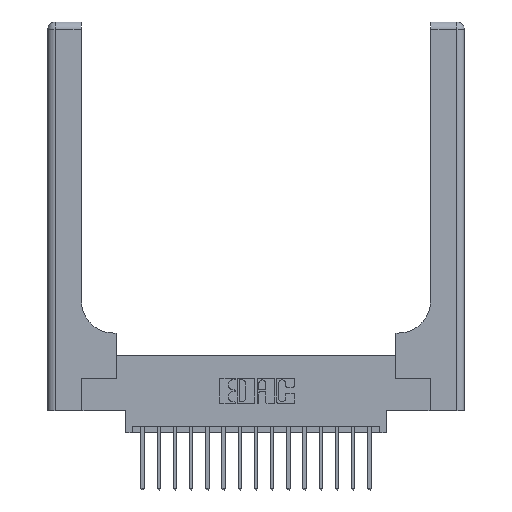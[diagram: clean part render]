
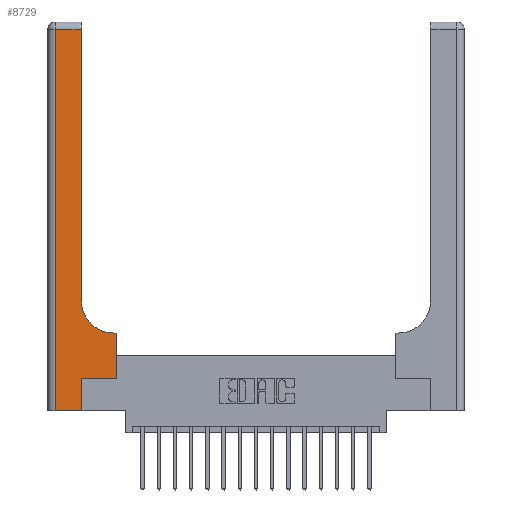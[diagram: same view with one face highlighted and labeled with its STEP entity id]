
A CAD part, top view. The second image highlights one B-rep face of the part: STEP entity #8729.
In plain terms, the highlighted planar face has unit normal (0, 0, 1).
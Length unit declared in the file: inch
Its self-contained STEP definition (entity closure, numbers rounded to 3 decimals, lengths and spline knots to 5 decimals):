
#74 = CARTESIAN_POINT ( 'NONE',  ( 0.06, 3., 0.37 ) ) ;
#119 = EDGE_CURVE ( 'NONE', #1267, #13343, #17823, .T. ) ;
#148 = DIRECTION ( 'NONE',  ( 1., 0., 0. ) ) ;
#470 = VERTEX_POINT ( 'NONE', #6315 ) ;
#1227 = VECTOR ( 'NONE', #5650, 39.37008 ) ;
#1267 = VERTEX_POINT ( 'NONE', #4174 ) ;
#1380 = ORIENTED_EDGE ( 'NONE', *, *, #119, .T. ) ;
#1852 = EDGE_CURVE ( 'NONE', #11906, #4479, #4620, .T. ) ;
#1927 = CARTESIAN_POINT ( 'NONE',  ( 0.528, 0.6, 0.37 ) ) ;
#1991 = EDGE_CURVE ( 'NONE', #9378, #11906, #12276, .T. ) ;
#2006 = CARTESIAN_POINT ( 'NONE',  ( 0.528, 0.25, 0.37 ) ) ;
#2130 = AXIS2_PLACEMENT_3D ( 'NONE', #5486, #17519, #5780 ) ;
#2336 = DIRECTION ( 'NONE',  ( -1., 0., 0. ) ) ;
#2388 = ORIENTED_EDGE ( 'NONE', *, *, #10496, .T. ) ;
#3662 = DIRECTION ( 'NONE',  ( 0., 0., -1. ) ) ;
#4174 = CARTESIAN_POINT ( 'NONE',  ( 0.06, 0., 0.37 ) ) ;
#4377 = VECTOR ( 'NONE', #17555, 39.37008 ) ;
#4388 = CARTESIAN_POINT ( 'NONE',  ( 0., 2.94, 0.37 ) ) ;
#4479 = VERTEX_POINT ( 'NONE', #1927 ) ;
#4620 = LINE ( 'NONE', #6002, #13927 ) ;
#4762 = CARTESIAN_POINT ( 'NONE',  ( 0.265, 0., 0.37 ) ) ;
#5486 = CARTESIAN_POINT ( 'NONE',  ( 0.51, 0.85, 0.37 ) ) ;
#5650 = DIRECTION ( 'NONE',  ( 0., 1., 0. ) ) ;
#5780 = DIRECTION ( 'NONE',  ( 1., 0., 0. ) ) ;
#5912 = DIRECTION ( 'NONE',  ( 0., 1., 0. ) ) ;
#6002 = CARTESIAN_POINT ( 'NONE',  ( 0.528, 0.25, 0.37 ) ) ;
#6315 = CARTESIAN_POINT ( 'NONE',  ( 0.51, 0.6, 0.37 ) ) ;
#6326 = VECTOR ( 'NONE', #6526, 39.37008 ) ;
#6526 = DIRECTION ( 'NONE',  ( 0., 1., 0. ) ) ;
#6713 = LINE ( 'NONE', #9716, #13799 ) ;
#6732 = ORIENTED_EDGE ( 'NONE', *, *, #9025, .T. ) ;
#7118 = CARTESIAN_POINT ( 'NONE',  ( 0.265, 0., 0.37 ) ) ;
#7294 = VECTOR ( 'NONE', #10831, 39.37008 ) ;
#7309 = LINE ( 'NONE', #4388, #19017 ) ;
#7503 = DIRECTION ( 'NONE',  ( -1., 0., 0. ) ) ;
#8395 = ORIENTED_EDGE ( 'NONE', *, *, #1991, .T. ) ;
#8627 = LINE ( 'NONE', #74, #4377 ) ;
#8729 = ADVANCED_FACE ( 'NONE', ( #18431 ), #15319, .F. ) ;
#8744 = VERTEX_POINT ( 'NONE', #14148 ) ;
#9025 = EDGE_CURVE ( 'NONE', #8744, #12203, #14755, .T. ) ;
#9360 = ORIENTED_EDGE ( 'NONE', *, *, #16383, .T. ) ;
#9378 = VERTEX_POINT ( 'NONE', #14448 ) ;
#9418 = EDGE_LOOP ( 'NONE', ( #6732, #16748, #2388, #1380, #16699, #8395, #17767, #9360, #15405 ) ) ;
#9716 = CARTESIAN_POINT ( 'NONE',  ( 0.26, 0.6, 0.37 ) ) ;
#10496 = EDGE_CURVE ( 'NONE', #16231, #1267, #8627, .T. ) ;
#10831 = DIRECTION ( 'NONE',  ( 1., 0., 0. ) ) ;
#11025 = CARTESIAN_POINT ( 'NONE',  ( 0.265, 0.25, 0.37 ) ) ;
#11906 = VERTEX_POINT ( 'NONE', #2006 ) ;
#12203 = VERTEX_POINT ( 'NONE', #14722 ) ;
#12231 = CARTESIAN_POINT ( 'NONE',  ( 0.06, 2.94, 0.37 ) ) ;
#12276 = LINE ( 'NONE', #11025, #7294 ) ;
#12354 = CIRCLE ( 'NONE', #2130, 0.25 ) ;
#13200 = CARTESIAN_POINT ( 'NONE',  ( 0.26, 3., 0.37 ) ) ;
#13343 = VERTEX_POINT ( 'NONE', #7118 ) ;
#13502 = EDGE_CURVE ( 'NONE', #12203, #16231, #7309, .T. ) ;
#13799 = VECTOR ( 'NONE', #2336, 39.37008 ) ;
#13851 = DIRECTION ( 'NONE',  ( -1., 0., 0. ) ) ;
#13874 = LINE ( 'NONE', #4762, #6326 ) ;
#13927 = VECTOR ( 'NONE', #5912, 39.37008 ) ;
#14148 = CARTESIAN_POINT ( 'NONE',  ( 0.26, 0.85, 0.37 ) ) ;
#14448 = CARTESIAN_POINT ( 'NONE',  ( 0.265, 0.25, 0.37 ) ) ;
#14580 = VECTOR ( 'NONE', #148, 39.37008 ) ;
#14722 = CARTESIAN_POINT ( 'NONE',  ( 0.26, 2.94, 0.37 ) ) ;
#14755 = LINE ( 'NONE', #13200, #1227 ) ;
#15260 = CARTESIAN_POINT ( 'NONE',  ( 0., 0., 0.37 ) ) ;
#15319 = PLANE ( 'NONE',  #15772 ) ;
#15405 = ORIENTED_EDGE ( 'NONE', *, *, #19181, .T. ) ;
#15613 = CARTESIAN_POINT ( 'NONE',  ( 0., 3., 0.37 ) ) ;
#15772 = AXIS2_PLACEMENT_3D ( 'NONE', #15613, #3662, #13851 ) ;
#16231 = VERTEX_POINT ( 'NONE', #12231 ) ;
#16277 = EDGE_CURVE ( 'NONE', #13343, #9378, #13874, .T. ) ;
#16383 = EDGE_CURVE ( 'NONE', #4479, #470, #6713, .T. ) ;
#16699 = ORIENTED_EDGE ( 'NONE', *, *, #16277, .T. ) ;
#16748 = ORIENTED_EDGE ( 'NONE', *, *, #13502, .T. ) ;
#17519 = DIRECTION ( 'NONE',  ( 0., 0., -1. ) ) ;
#17555 = DIRECTION ( 'NONE',  ( 0., -1., 0. ) ) ;
#17767 = ORIENTED_EDGE ( 'NONE', *, *, #1852, .T. ) ;
#17823 = LINE ( 'NONE', #15260, #14580 ) ;
#18431 = FACE_OUTER_BOUND ( 'NONE', #9418, .T. ) ;
#19017 = VECTOR ( 'NONE', #7503, 39.37008 ) ;
#19181 = EDGE_CURVE ( 'NONE', #470, #8744, #12354, .T. ) ;
